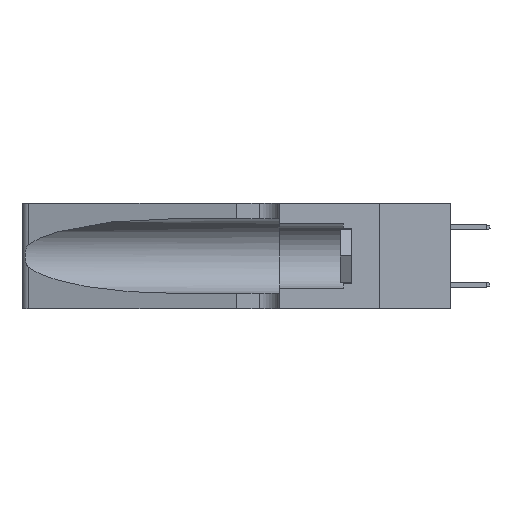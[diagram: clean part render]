
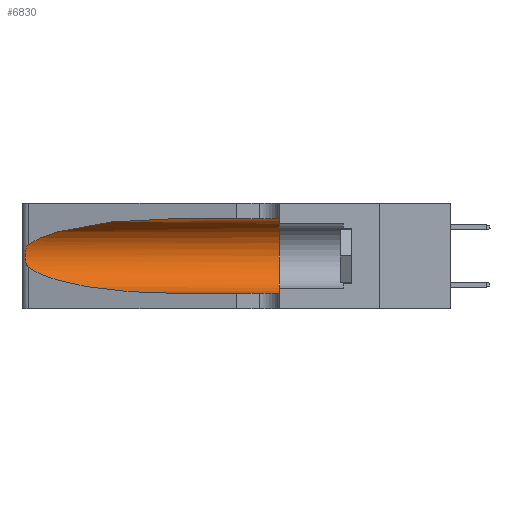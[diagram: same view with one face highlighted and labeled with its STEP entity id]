
A CAD part, left-side view. The second image highlights one B-rep face of the part: STEP entity #6830.
In plain terms, the highlighted cylindrical face has radius 3.308 mm (diameter 6.617 mm), a partial arc.
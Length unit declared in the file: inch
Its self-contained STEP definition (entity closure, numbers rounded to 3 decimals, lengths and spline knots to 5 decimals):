
#1457 = CARTESIAN_POINT ( 'NONE',  ( 0.25487, 1.22718, 0.22369 ) ) ;
#1671 = CARTESIAN_POINT ( 'NONE',  ( 0.26018, 1.23835, 0.19895 ) ) ;
#2383 = DIRECTION ( 'NONE',  ( 0., -1., 0. ) ) ;
#3838 = FACE_OUTER_BOUND ( 'NONE', #7675, .T. ) ;
#4645 = CARTESIAN_POINT ( 'NONE',  ( 0.26075, 1.23896, 0.178 ) ) ;
#5558 = CARTESIAN_POINT ( 'NONE',  ( 0.1305, 1.61858, 0.05475 ) ) ;
#6009 = CIRCLE ( 'NONE', #23535, 0.13025 ) ;
#6218 = CARTESIAN_POINT ( 'NONE',  ( 0.1305, 0.35, 0.31525 ) ) ;
#6830 = ADVANCED_FACE ( 'NONE', ( #3838 ), #26438, .F. ) ;
#7438 = CARTESIAN_POINT ( 'NONE',  ( 0.1305, 1.61858, 0.185 ) ) ;
#7595 = CARTESIAN_POINT ( 'NONE',  ( 0.25854, 1.2359, 0.20912 ) ) ;
#7675 = EDGE_LOOP ( 'NONE', ( #15374, #13118, #37577, #33570, #38164, #12038 ) ) ;
#7814 = CARTESIAN_POINT ( 'NONE',  ( 0.1305, 1.61858, 0.31525 ) ) ;
#9354 = EDGE_CURVE ( 'NONE', #24772, #14899, #6009, .T. ) ;
#10366 = DIRECTION ( 'NONE',  ( 0., -1., 0. ) ) ;
#10782 = CARTESIAN_POINT ( 'NONE',  ( 0.25555, 1.22994, 0.2215 ) ) ;
#10982 = CARTESIAN_POINT ( 'NONE',  ( 0.25856, 1.23593, 0.16098 ) ) ;
#11103 = CARTESIAN_POINT ( 'NONE',  ( 0.1305, 0.72297, 0.05475 ) ) ;
#11192 = CARTESIAN_POINT ( 'NONE',  ( 0.26017, 1.23833, 0.17102 ) ) ;
#12038 = ORIENTED_EDGE ( 'NONE', *, *, #12444, .F. ) ;
#12444 = EDGE_CURVE ( 'NONE', #39381, #24772, #26834, .T. ) ;
#13118 = ORIENTED_EDGE ( 'NONE', *, *, #28226, .T. ) ;
#13230 = CARTESIAN_POINT ( 'NONE',  ( 0.2373, 1.15595, 0.28018 ) ) ;
#14377 = CARTESIAN_POINT ( 'NONE',  ( 0.25789, 1.23486, 0.15765 ) ) ;
#14899 = VERTEX_POINT ( 'NONE', #20683 ) ;
#14975 = CARTESIAN_POINT ( 'NONE',  ( 0.1305, 0.72297, 0.05475 ) ) ;
#15019 = B_SPLINE_CURVE_WITH_KNOTS ( 'NONE', 3,
 ( #1457, #10782, #23649, #17355, #7595, #1671, #26607, #4645, #11192, #10982, #14377, #33791, #24057, #30215 ),
 .UNSPECIFIED., .F., .F.,
 ( 4, 2, 2, 2, 2, 2, 4 ),
 ( 0., 0.00027, 0.00053, 0.00107, 0.0016, 0.00187, 0.00214 ),
 .UNSPECIFIED. ) ;
#15039 = EDGE_CURVE ( 'NONE', #34940, #36266, #39653, .T. ) ;
#15374 = ORIENTED_EDGE ( 'NONE', *, *, #37431, .T. ) ;
#17179 = DIRECTION ( 'NONE',  ( 0., 0., -1. ) ) ;
#17355 = CARTESIAN_POINT ( 'NONE',  ( 0.25787, 1.23484, 0.2124 ) ) ;
#18133 = CARTESIAN_POINT ( 'NONE',  ( 0.25487, 1.22718, 0.14631 ) ) ;
#20329 = DIRECTION ( 'NONE',  ( 0., -1., 0. ) ) ;
#20683 = CARTESIAN_POINT ( 'NONE',  ( 0.1305, 0.35, 0.05475 ) ) ;
#21470 = CARTESIAN_POINT ( 'NONE',  ( 0.1305, 0.35, 0.185 ) ) ;
#21610 = LINE ( 'NONE', #5558, #39512 ) ;
#23535 = AXIS2_PLACEMENT_3D ( 'NONE', #21470, #34367, #31180 ) ;
#23649 = CARTESIAN_POINT ( 'NONE',  ( 0.25639, 1.23184, 0.21858 ) ) ;
#24057 = CARTESIAN_POINT ( 'NONE',  ( 0.25555, 1.22993, 0.14849 ) ) ;
#24165 = AXIS2_PLACEMENT_3D ( 'NONE', #7438, #20329, #17179 ) ;
#24772 = VERTEX_POINT ( 'NONE', #6218 ) ;
#26103 = CARTESIAN_POINT ( 'NONE',  ( 0.25487, 1.22718, 0.22369 ) ) ;
#26438 = CYLINDRICAL_SURFACE ( 'NONE', #24165, 0.13025 ) ;
#26515 = EDGE_CURVE ( 'NONE', #36266, #14899, #21610, .T. ) ;
#26607 = CARTESIAN_POINT ( 'NONE',  ( 0.26075, 1.23896, 0.19203 ) ) ;
#26737 = CARTESIAN_POINT ( 'NONE',  ( 0.18966, 0.96281, 0.31525 ) ) ;
#26834 = LINE ( 'NONE', #7814, #33443 ) ;
#27722 = CARTESIAN_POINT ( 'NONE',  ( 0.1305, 0.72297, 0.31525 ) ) ;
#28226 = EDGE_CURVE ( 'NONE', #28254, #34940, #15019, .T. ) ;
#28254 = VERTEX_POINT ( 'NONE', #30413 ) ;
#29906 = CARTESIAN_POINT ( 'NONE',  ( 0.1305, 0.72297, 0.31525 ) ) ;
#30215 = CARTESIAN_POINT ( 'NONE',  ( 0.25487, 1.22718, 0.14631 ) ) ;
#30413 = CARTESIAN_POINT ( 'NONE',  ( 0.25487, 1.22718, 0.22369 ) ) ;
#31013 = CARTESIAN_POINT ( 'NONE',  ( 0.2373, 1.15595, 0.08982 ) ) ;
#31180 = DIRECTION ( 'NONE',  ( 0., 0., 1. ) ) ;
#33443 = VECTOR ( 'NONE', #10366, 39.37008 ) ;
#33570 = ORIENTED_EDGE ( 'NONE', *, *, #26515, .T. ) ;
#33791 = CARTESIAN_POINT ( 'NONE',  ( 0.25639, 1.23186, 0.15144 ) ) ;
#34367 = DIRECTION ( 'NONE',  ( 0., 1., 0. ) ) ;
#34940 = VERTEX_POINT ( 'NONE', #41482 ) ;
#36266 = VERTEX_POINT ( 'NONE', #11103 ) ;
#37431 = EDGE_CURVE ( 'NONE', #39381, #28254, #38551, .T. ) ;
#37577 = ORIENTED_EDGE ( 'NONE', *, *, #15039, .T. ) ;
#37762 = CARTESIAN_POINT ( 'NONE',  ( 0.18966, 0.96281, 0.05475 ) ) ;
#38164 = ORIENTED_EDGE ( 'NONE', *, *, #9354, .F. ) ;
#38551 =( BOUNDED_CURVE ( )  B_SPLINE_CURVE ( 3, ( #29906, #26737, #13230, #26103 ),
 .UNSPECIFIED., .F., .F. ) 
 B_SPLINE_CURVE_WITH_KNOTS ( ( 4, 4 ),
 ( 1.5708, 2.84003 ),
 .UNSPECIFIED. ) 
 CURVE ( )  GEOMETRIC_REPRESENTATION_ITEM ( )  RATIONAL_B_SPLINE_CURVE ( ( 1., 0.87, 0.87, 1. ) ) 
 REPRESENTATION_ITEM ( '' )  );
#39381 = VERTEX_POINT ( 'NONE', #27722 ) ;
#39512 = VECTOR ( 'NONE', #2383, 39.37008 ) ;
#39653 =( BOUNDED_CURVE ( )  B_SPLINE_CURVE ( 3, ( #18133, #31013, #37762, #14975 ),
 .UNSPECIFIED., .F., .F. ) 
 B_SPLINE_CURVE_WITH_KNOTS ( ( 4, 4 ),
 ( 3.44316, 4.71239 ),
 .UNSPECIFIED. ) 
 CURVE ( )  GEOMETRIC_REPRESENTATION_ITEM ( )  RATIONAL_B_SPLINE_CURVE ( ( 1., 0.87, 0.87, 1. ) ) 
 REPRESENTATION_ITEM ( '' )  );
#41482 = CARTESIAN_POINT ( 'NONE',  ( 0.25487, 1.22718, 0.14631 ) ) ;
